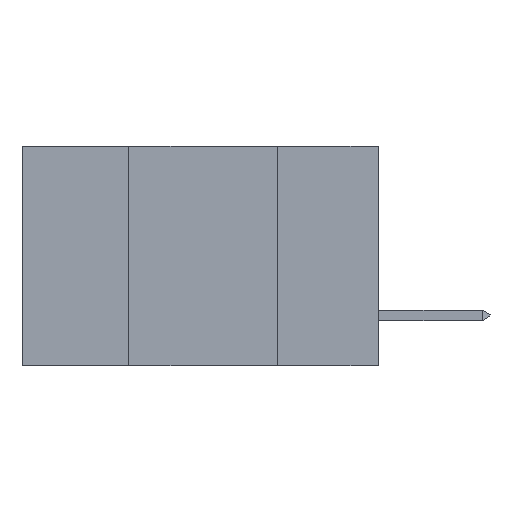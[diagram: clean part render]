
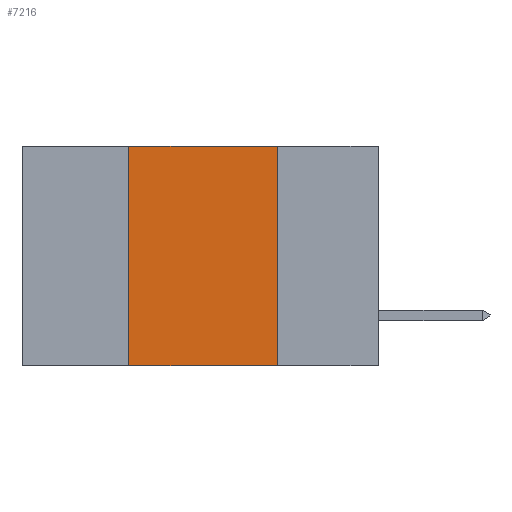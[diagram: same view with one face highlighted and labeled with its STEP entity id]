
A CAD part, left-side view. The second image highlights one B-rep face of the part: STEP entity #7216.
In plain terms, the highlighted planar face has unit normal (-1, 0, 0).
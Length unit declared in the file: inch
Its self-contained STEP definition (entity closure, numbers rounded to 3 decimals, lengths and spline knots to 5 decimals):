
#163 = LINE ( 'NONE', #6719, #584 ) ;
#221 = ORIENTED_EDGE ( 'NONE', *, *, #11552, .F. ) ;
#584 = VECTOR ( 'NONE', #1363, 39.37008 ) ;
#1363 = DIRECTION ( 'NONE',  ( 0., 0., 1. ) ) ;
#1371 = CARTESIAN_POINT ( 'NONE',  ( 0., 0.6, -0.37 ) ) ;
#2323 = EDGE_CURVE ( 'NONE', #11694, #8080, #13041, .T. ) ;
#2868 = VECTOR ( 'NONE', #11834, 39.37008 ) ;
#3478 = EDGE_CURVE ( 'NONE', #6034, #11694, #13909, .T. ) ;
#3652 = DIRECTION ( 'NONE',  ( 0., -1., 0. ) ) ;
#4112 = CARTESIAN_POINT ( 'NONE',  ( 0., 0.6, 0. ) ) ;
#4344 = EDGE_LOOP ( 'NONE', ( #6376, #11936, #221, #12087 ) ) ;
#4394 = CARTESIAN_POINT ( 'NONE',  ( 0., 0.17, -0.37 ) ) ;
#4578 = LINE ( 'NONE', #1371, #8716 ) ;
#6034 = VERTEX_POINT ( 'NONE', #6866 ) ;
#6038 = DIRECTION ( 'NONE',  ( 0., -1., 0. ) ) ;
#6376 = ORIENTED_EDGE ( 'NONE', *, *, #2323, .F. ) ;
#6464 = CARTESIAN_POINT ( 'NONE',  ( 0., 0.17, -0.37 ) ) ;
#6591 = FACE_OUTER_BOUND ( 'NONE', #4344, .T. ) ;
#6719 = CARTESIAN_POINT ( 'NONE',  ( 0., 0.42, -0.37 ) ) ;
#6866 = CARTESIAN_POINT ( 'NONE',  ( 0., 0.42, 0. ) ) ;
#6930 = DIRECTION ( 'NONE',  ( 1., 0., 0. ) ) ;
#7216 = ADVANCED_FACE ( 'NONE', ( #6591 ), #10938, .F. ) ;
#7220 = EDGE_CURVE ( 'NONE', #12051, #8080, #4578, .T. ) ;
#8080 = VERTEX_POINT ( 'NONE', #4394 ) ;
#8138 = CARTESIAN_POINT ( 'NONE',  ( 0., 0.17, 0. ) ) ;
#8426 = VECTOR ( 'NONE', #6038, 39.37008 ) ;
#8716 = VECTOR ( 'NONE', #3652, 39.37008 ) ;
#8801 = CARTESIAN_POINT ( 'NONE',  ( 0., 0.6, 0. ) ) ;
#9263 = CARTESIAN_POINT ( 'NONE',  ( 0., 0.42, -0.37 ) ) ;
#9404 = AXIS2_PLACEMENT_3D ( 'NONE', #8801, #6930, #11009 ) ;
#10938 = PLANE ( 'NONE',  #9404 ) ;
#11009 = DIRECTION ( 'NONE',  ( 0., 0., -1. ) ) ;
#11552 = EDGE_CURVE ( 'NONE', #12051, #6034, #163, .T. ) ;
#11694 = VERTEX_POINT ( 'NONE', #8138 ) ;
#11834 = DIRECTION ( 'NONE',  ( 0., 0., -1. ) ) ;
#11936 = ORIENTED_EDGE ( 'NONE', *, *, #3478, .F. ) ;
#12051 = VERTEX_POINT ( 'NONE', #9263 ) ;
#12087 = ORIENTED_EDGE ( 'NONE', *, *, #7220, .T. ) ;
#13041 = LINE ( 'NONE', #6464, #2868 ) ;
#13909 = LINE ( 'NONE', #4112, #8426 ) ;
